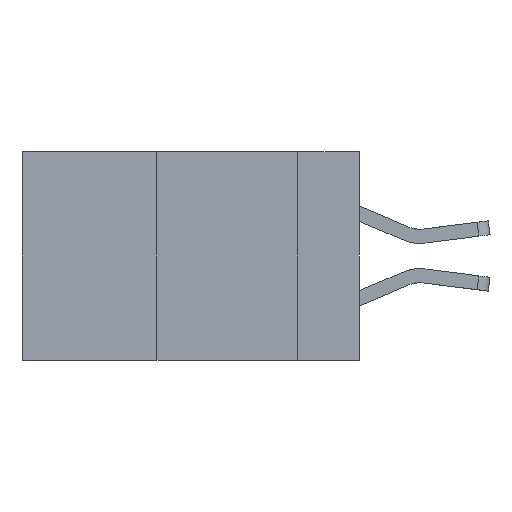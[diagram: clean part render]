
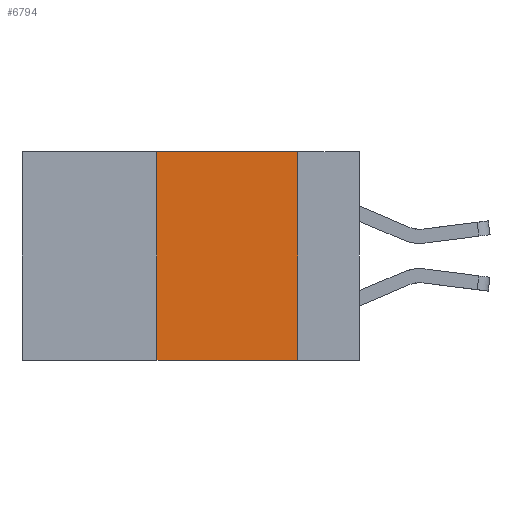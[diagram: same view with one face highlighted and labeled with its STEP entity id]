
A CAD part, left-side view. The second image highlights one B-rep face of the part: STEP entity #6794.
In plain terms, the highlighted planar face has unit normal (-1, 0, 0).
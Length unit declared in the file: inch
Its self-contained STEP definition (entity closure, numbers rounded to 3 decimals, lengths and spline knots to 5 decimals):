
#125 = LINE ( 'NONE', #5148, #4662 ) ;
#261 = CARTESIAN_POINT ( 'NONE',  ( 0., 0.36, -0.37 ) ) ;
#457 = VECTOR ( 'NONE', #3693, 39.37008 ) ;
#613 = VECTOR ( 'NONE', #11173, 39.37008 ) ;
#934 = LINE ( 'NONE', #10382, #613 ) ;
#1596 = LINE ( 'NONE', #6405, #5940 ) ;
#2989 = AXIS2_PLACEMENT_3D ( 'NONE', #6131, #8805, #3619 ) ;
#3446 = ORIENTED_EDGE ( 'NONE', *, *, #10118, .F. ) ;
#3526 = LINE ( 'NONE', #6241, #457 ) ;
#3619 = DIRECTION ( 'NONE',  ( 0., 0., -1. ) ) ;
#3622 = ORIENTED_EDGE ( 'NONE', *, *, #10949, .F. ) ;
#3650 = ORIENTED_EDGE ( 'NONE', *, *, #7476, .F. ) ;
#3683 = CARTESIAN_POINT ( 'NONE',  ( 0., 0.11, -0.37 ) ) ;
#3688 = ORIENTED_EDGE ( 'NONE', *, *, #6253, .T. ) ;
#3693 = DIRECTION ( 'NONE',  ( 0., -1., 0. ) ) ;
#4133 = FACE_OUTER_BOUND ( 'NONE', #9738, .T. ) ;
#4662 = VECTOR ( 'NONE', #6029, 39.37008 ) ;
#5053 = CARTESIAN_POINT ( 'NONE',  ( 0., 0.36, 0. ) ) ;
#5148 = CARTESIAN_POINT ( 'NONE',  ( 0., 0.6, 0. ) ) ;
#5935 = VERTEX_POINT ( 'NONE', #261 ) ;
#5940 = VECTOR ( 'NONE', #7347, 39.37008 ) ;
#6029 = DIRECTION ( 'NONE',  ( 0., -1., 0. ) ) ;
#6131 = CARTESIAN_POINT ( 'NONE',  ( 0., 0.6, 0. ) ) ;
#6241 = CARTESIAN_POINT ( 'NONE',  ( 0., 0.6, -0.37 ) ) ;
#6253 = EDGE_CURVE ( 'NONE', #5935, #8952, #3526, .T. ) ;
#6405 = CARTESIAN_POINT ( 'NONE',  ( 0., 0.36, 0. ) ) ;
#6794 = ADVANCED_FACE ( 'NONE', ( #4133 ), #7926, .F. ) ;
#7250 = VERTEX_POINT ( 'NONE', #8690 ) ;
#7347 = DIRECTION ( 'NONE',  ( 0., 0., 1. ) ) ;
#7476 = EDGE_CURVE ( 'NONE', #5935, #10022, #1596, .T. ) ;
#7926 = PLANE ( 'NONE',  #2989 ) ;
#8690 = CARTESIAN_POINT ( 'NONE',  ( 0., 0.11, 0. ) ) ;
#8805 = DIRECTION ( 'NONE',  ( 1., 0., 0. ) ) ;
#8952 = VERTEX_POINT ( 'NONE', #3683 ) ;
#9738 = EDGE_LOOP ( 'NONE', ( #3446, #3622, #3650, #3688 ) ) ;
#10022 = VERTEX_POINT ( 'NONE', #5053 ) ;
#10118 = EDGE_CURVE ( 'NONE', #7250, #8952, #934, .T. ) ;
#10382 = CARTESIAN_POINT ( 'NONE',  ( 0., 0.11, 0. ) ) ;
#10949 = EDGE_CURVE ( 'NONE', #10022, #7250, #125, .T. ) ;
#11173 = DIRECTION ( 'NONE',  ( 0., 0., -1. ) ) ;
